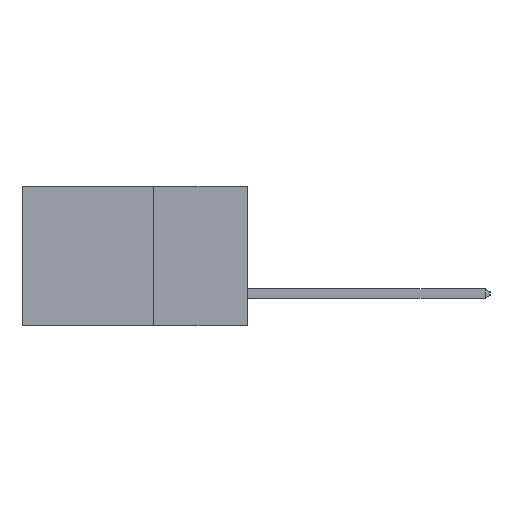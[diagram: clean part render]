
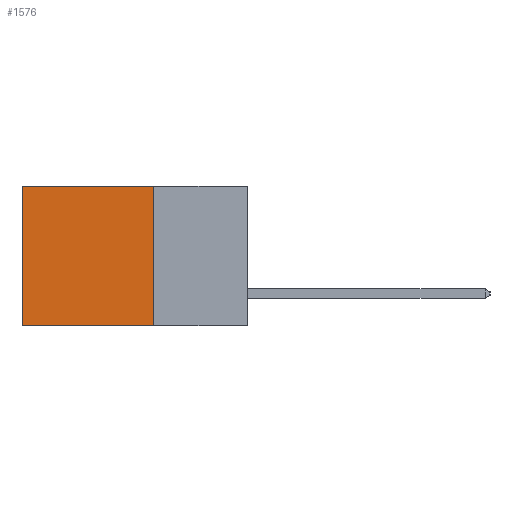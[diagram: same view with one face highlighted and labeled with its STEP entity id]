
A CAD part, left-side view. The second image highlights one B-rep face of the part: STEP entity #1576.
In plain terms, the highlighted planar face has unit normal (-1, 0, 0).
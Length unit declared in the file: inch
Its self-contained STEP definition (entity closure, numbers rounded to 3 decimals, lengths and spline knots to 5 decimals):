
#16 = VERTEX_POINT ( 'NONE', #15340 ) ;
#521 = DIRECTION ( 'NONE',  ( 0., 1., 0. ) ) ;
#1576 = ADVANCED_FACE ( 'NONE', ( #10931 ), #6733, .F. ) ;
#1740 = VECTOR ( 'NONE', #521, 39.37008 ) ;
#2412 = CARTESIAN_POINT ( 'NONE',  ( 0.298, 0.25, 0. ) ) ;
#2593 = VECTOR ( 'NONE', #13693, 39.37008 ) ;
#2701 = DIRECTION ( 'NONE',  ( 0., 0., -1. ) ) ;
#3808 = LINE ( 'NONE', #14604, #10454 ) ;
#4184 = VERTEX_POINT ( 'NONE', #7627 ) ;
#4244 = CARTESIAN_POINT ( 'NONE',  ( 0.298, 0.25, -0.37 ) ) ;
#4783 = DIRECTION ( 'NONE',  ( 0., 0., -1. ) ) ;
#4948 = DIRECTION ( 'NONE',  ( 1., 0., 0. ) ) ;
#4988 = CARTESIAN_POINT ( 'NONE',  ( 0.298, 0.25, 0. ) ) ;
#5273 = CARTESIAN_POINT ( 'NONE',  ( 0.298, 0.6, 0. ) ) ;
#5987 = VECTOR ( 'NONE', #2701, 39.37008 ) ;
#6556 = EDGE_LOOP ( 'NONE', ( #10630, #8602, #13581, #14905 ) ) ;
#6733 = PLANE ( 'NONE',  #7527 ) ;
#6822 = EDGE_CURVE ( 'NONE', #9630, #8190, #16706, .T. ) ;
#7527 = AXIS2_PLACEMENT_3D ( 'NONE', #4988, #4948, #4783 ) ;
#7627 = CARTESIAN_POINT ( 'NONE',  ( 0.298, 0.6, -0.37 ) ) ;
#7804 = EDGE_CURVE ( 'NONE', #9630, #16, #3808, .T. ) ;
#8190 = VERTEX_POINT ( 'NONE', #4244 ) ;
#8431 = CARTESIAN_POINT ( 'NONE',  ( 0.298, 0.25, -0.37 ) ) ;
#8602 = ORIENTED_EDGE ( 'NONE', *, *, #13146, .F. ) ;
#8777 = LINE ( 'NONE', #8431, #1740 ) ;
#9513 = LINE ( 'NONE', #5273, #5987 ) ;
#9630 = VERTEX_POINT ( 'NONE', #2412 ) ;
#9773 = EDGE_CURVE ( 'NONE', #16, #4184, #9513, .T. ) ;
#10454 = VECTOR ( 'NONE', #14003, 39.37008 ) ;
#10630 = ORIENTED_EDGE ( 'NONE', *, *, #9773, .T. ) ;
#10931 = FACE_OUTER_BOUND ( 'NONE', #6556, .T. ) ;
#13146 = EDGE_CURVE ( 'NONE', #8190, #4184, #8777, .T. ) ;
#13581 = ORIENTED_EDGE ( 'NONE', *, *, #6822, .F. ) ;
#13693 = DIRECTION ( 'NONE',  ( 0., 0., -1. ) ) ;
#14003 = DIRECTION ( 'NONE',  ( 0., 1., 0. ) ) ;
#14604 = CARTESIAN_POINT ( 'NONE',  ( 0.298, 0.25, 0. ) ) ;
#14905 = ORIENTED_EDGE ( 'NONE', *, *, #7804, .T. ) ;
#15340 = CARTESIAN_POINT ( 'NONE',  ( 0.298, 0.6, 0. ) ) ;
#15581 = CARTESIAN_POINT ( 'NONE',  ( 0.298, 0.25, 0. ) ) ;
#16706 = LINE ( 'NONE', #15581, #2593 ) ;
